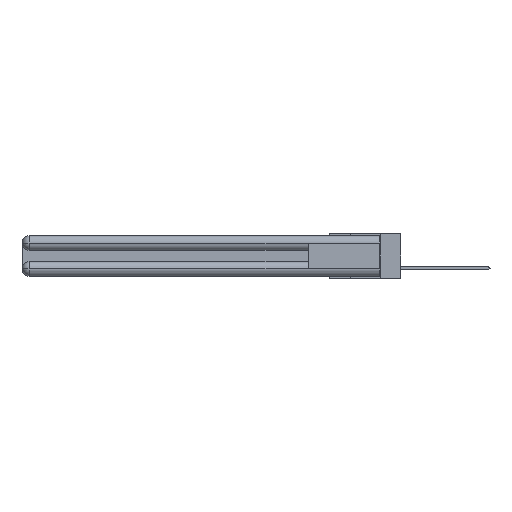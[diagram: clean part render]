
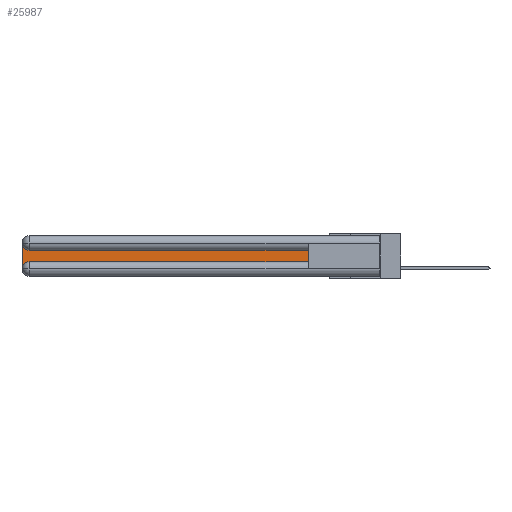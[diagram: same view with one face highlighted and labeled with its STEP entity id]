
A CAD part, left-side view. The second image highlights one B-rep face of the part: STEP entity #25987.
In plain terms, the highlighted planar face has unit normal (-1, 0, 0).
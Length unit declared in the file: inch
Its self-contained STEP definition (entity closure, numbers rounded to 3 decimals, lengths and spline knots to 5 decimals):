
#732 = VECTOR ( 'NONE', #18740, 39.37008 ) ;
#780 = CARTESIAN_POINT ( 'NONE',  ( 0.075, 0.6, -0.2175 ) ) ;
#1671 = EDGE_CURVE ( 'NONE', #22317, #7226, #19324, .T. ) ;
#1760 = ORIENTED_EDGE ( 'NONE', *, *, #23432, .T. ) ;
#2182 = DIRECTION ( 'NONE',  ( 0., -1., 0. ) ) ;
#2844 = ORIENTED_EDGE ( 'NONE', *, *, #1671, .T. ) ;
#3596 = CARTESIAN_POINT ( 'NONE',  ( 0.075, 2.94, -0.1225 ) ) ;
#4744 = CIRCLE ( 'NONE', #21820, 0.06 ) ;
#4777 = ORIENTED_EDGE ( 'NONE', *, *, #14637, .T. ) ;
#6130 = VECTOR ( 'NONE', #2182, 39.37008 ) ;
#6960 = EDGE_CURVE ( 'NONE', #7226, #25766, #11977, .T. ) ;
#7226 = VERTEX_POINT ( 'NONE', #27153 ) ;
#7317 = LINE ( 'NONE', #13665, #7994 ) ;
#7537 = VERTEX_POINT ( 'NONE', #8379 ) ;
#7994 = VECTOR ( 'NONE', #24545, 39.37008 ) ;
#8379 = CARTESIAN_POINT ( 'NONE',  ( 0.075, 3., -0.0625 ) ) ;
#8723 = CARTESIAN_POINT ( 'NONE',  ( 0.075, 3., -0.2775 ) ) ;
#9234 = FACE_OUTER_BOUND ( 'NONE', #28495, .T. ) ;
#10345 = CARTESIAN_POINT ( 'NONE',  ( 0.075, 0.6, -0.1225 ) ) ;
#10742 = CARTESIAN_POINT ( 'NONE',  ( 0.075, 2.94, -0.2775 ) ) ;
#11387 = AXIS2_PLACEMENT_3D ( 'NONE', #15320, #12988, #24251 ) ;
#11787 = DIRECTION ( 'NONE',  ( 1., 0., 0. ) ) ;
#11977 = LINE ( 'NONE', #24090, #6130 ) ;
#12361 = DIRECTION ( 'NONE',  ( 0., 0., -1. ) ) ;
#12737 = DIRECTION ( 'NONE',  ( 1., 0., 0. ) ) ;
#12988 = DIRECTION ( 'NONE',  ( 1., 0., 0. ) ) ;
#13665 = CARTESIAN_POINT ( 'NONE',  ( 0.075, 3., -0.2175 ) ) ;
#14028 = VECTOR ( 'NONE', #25364, 39.37008 ) ;
#14233 = VERTEX_POINT ( 'NONE', #3596 ) ;
#14494 = LINE ( 'NONE', #780, #732 ) ;
#14637 = EDGE_CURVE ( 'NONE', #7537, #22317, #7317, .T. ) ;
#15320 = CARTESIAN_POINT ( 'NONE',  ( 0.075, 3., -0.1225 ) ) ;
#16190 = CARTESIAN_POINT ( 'NONE',  ( 0.075, 0.6, -0.2175 ) ) ;
#17622 = PLANE ( 'NONE',  #11387 ) ;
#18740 = DIRECTION ( 'NONE',  ( 0., 0., 1. ) ) ;
#19324 = CIRCLE ( 'NONE', #26975, 0.06 ) ;
#21820 = AXIS2_PLACEMENT_3D ( 'NONE', #25640, #12737, #12361 ) ;
#22317 = VERTEX_POINT ( 'NONE', #8723 ) ;
#22740 = DIRECTION ( 'NONE',  ( 0., 0., -1. ) ) ;
#23381 = EDGE_CURVE ( 'NONE', #28425, #14233, #25722, .T. ) ;
#23432 = EDGE_CURVE ( 'NONE', #14233, #7537, #4744, .T. ) ;
#24039 = ORIENTED_EDGE ( 'NONE', *, *, #23381, .T. ) ;
#24090 = CARTESIAN_POINT ( 'NONE',  ( 0.075, 0.6, -0.2175 ) ) ;
#24251 = DIRECTION ( 'NONE',  ( 0., 0., -1. ) ) ;
#24513 = ORIENTED_EDGE ( 'NONE', *, *, #24555, .T. ) ;
#24545 = DIRECTION ( 'NONE',  ( 0., 0., -1. ) ) ;
#24555 = EDGE_CURVE ( 'NONE', #25766, #28425, #14494, .T. ) ;
#25364 = DIRECTION ( 'NONE',  ( 0., 1., 0. ) ) ;
#25640 = CARTESIAN_POINT ( 'NONE',  ( 0.075, 2.94, -0.0625 ) ) ;
#25658 = CARTESIAN_POINT ( 'NONE',  ( 0.075, 0.6, -0.1225 ) ) ;
#25722 = LINE ( 'NONE', #25658, #14028 ) ;
#25729 = ORIENTED_EDGE ( 'NONE', *, *, #6960, .T. ) ;
#25766 = VERTEX_POINT ( 'NONE', #16190 ) ;
#25987 = ADVANCED_FACE ( 'NONE', ( #9234 ), #17622, .F. ) ;
#26975 = AXIS2_PLACEMENT_3D ( 'NONE', #10742, #11787, #22740 ) ;
#27153 = CARTESIAN_POINT ( 'NONE',  ( 0.075, 2.94, -0.2175 ) ) ;
#28425 = VERTEX_POINT ( 'NONE', #10345 ) ;
#28495 = EDGE_LOOP ( 'NONE', ( #24039, #1760, #4777, #2844, #25729, #24513 ) ) ;
